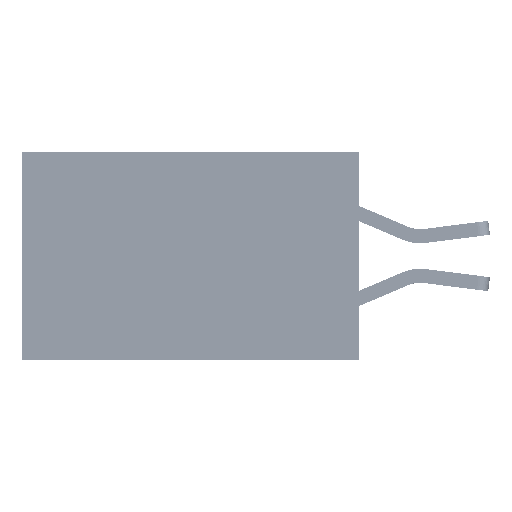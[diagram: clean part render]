
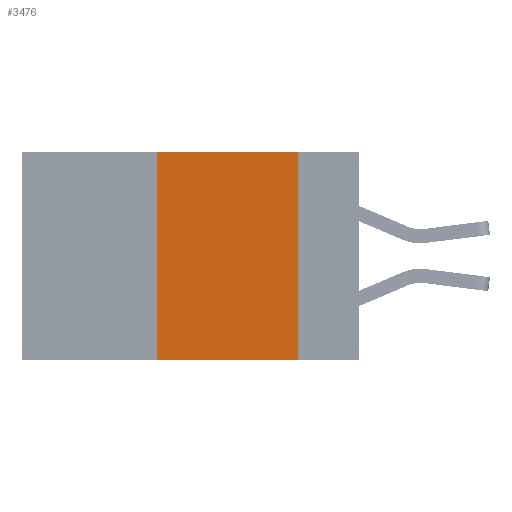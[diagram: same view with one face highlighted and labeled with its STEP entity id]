
A CAD part, left-side view. The second image highlights one B-rep face of the part: STEP entity #3476.
In plain terms, the highlighted planar face has unit normal (-1, 0, 0).
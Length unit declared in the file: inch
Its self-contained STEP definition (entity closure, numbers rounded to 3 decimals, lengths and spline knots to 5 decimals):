
#2808 = CARTESIAN_POINT ( 'NONE',  ( 0., 0.11, 0. ) ) ;
#3185 = VECTOR ( 'NONE', #15512, 39.37008 ) ;
#3476 = ADVANCED_FACE ( 'NONE', ( #34048 ), #12711, .F. ) ;
#9123 = EDGE_LOOP ( 'NONE', ( #38714, #12974, #18870, #16122 ) ) ;
#11270 = DIRECTION ( 'NONE',  ( 0., 0., -1. ) ) ;
#11977 = VERTEX_POINT ( 'NONE', #2808 ) ;
#12711 = PLANE ( 'NONE',  #16600 ) ;
#12974 = ORIENTED_EDGE ( 'NONE', *, *, #14945, .F. ) ;
#13414 = LINE ( 'NONE', #42507, #3185 ) ;
#14846 = VERTEX_POINT ( 'NONE', #23472 ) ;
#14945 = EDGE_CURVE ( 'NONE', #37247, #11977, #35067, .T. ) ;
#15512 = DIRECTION ( 'NONE',  ( 0., 0., 1. ) ) ;
#16122 = ORIENTED_EDGE ( 'NONE', *, *, #39440, .T. ) ;
#16144 = VECTOR ( 'NONE', #11270, 39.37008 ) ;
#16600 = AXIS2_PLACEMENT_3D ( 'NONE', #34648, #39499, #43377 ) ;
#17596 = LINE ( 'NONE', #23565, #30755 ) ;
#18870 = ORIENTED_EDGE ( 'NONE', *, *, #39445, .F. ) ;
#19873 = CARTESIAN_POINT ( 'NONE',  ( 0., 0.11, -0.37 ) ) ;
#20262 = CARTESIAN_POINT ( 'NONE',  ( 0., 0.6, 0. ) ) ;
#22086 = EDGE_CURVE ( 'NONE', #11977, #48750, #45581, .T. ) ;
#23336 = CARTESIAN_POINT ( 'NONE',  ( 0., 0.11, 0. ) ) ;
#23472 = CARTESIAN_POINT ( 'NONE',  ( 0., 0.36, -0.37 ) ) ;
#23565 = CARTESIAN_POINT ( 'NONE',  ( 0., 0.6, -0.37 ) ) ;
#26113 = VECTOR ( 'NONE', #39191, 39.37008 ) ;
#30755 = VECTOR ( 'NONE', #46232, 39.37008 ) ;
#34048 = FACE_OUTER_BOUND ( 'NONE', #9123, .T. ) ;
#34648 = CARTESIAN_POINT ( 'NONE',  ( 0., 0.6, 0. ) ) ;
#35067 = LINE ( 'NONE', #20262, #26113 ) ;
#37247 = VERTEX_POINT ( 'NONE', #47109 ) ;
#38714 = ORIENTED_EDGE ( 'NONE', *, *, #22086, .F. ) ;
#39191 = DIRECTION ( 'NONE',  ( 0., -1., 0. ) ) ;
#39440 = EDGE_CURVE ( 'NONE', #14846, #48750, #17596, .T. ) ;
#39445 = EDGE_CURVE ( 'NONE', #14846, #37247, #13414, .T. ) ;
#39499 = DIRECTION ( 'NONE',  ( 1., 0., 0. ) ) ;
#42507 = CARTESIAN_POINT ( 'NONE',  ( 0., 0.36, 0. ) ) ;
#43377 = DIRECTION ( 'NONE',  ( 0., 0., -1. ) ) ;
#45581 = LINE ( 'NONE', #23336, #16144 ) ;
#46232 = DIRECTION ( 'NONE',  ( 0., -1., 0. ) ) ;
#47109 = CARTESIAN_POINT ( 'NONE',  ( 0., 0.36, 0. ) ) ;
#48750 = VERTEX_POINT ( 'NONE', #19873 ) ;
